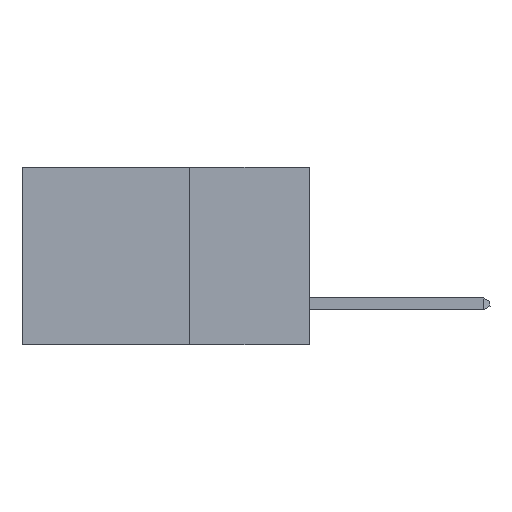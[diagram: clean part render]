
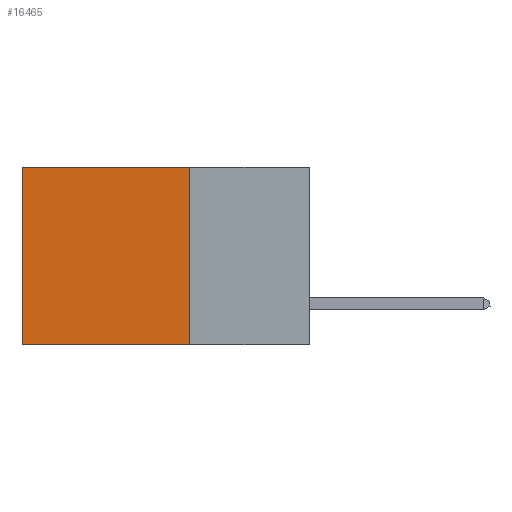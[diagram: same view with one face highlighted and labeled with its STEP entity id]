
A CAD part, left-side view. The second image highlights one B-rep face of the part: STEP entity #16465.
In plain terms, the highlighted planar face has unit normal (-1, 0, 0).
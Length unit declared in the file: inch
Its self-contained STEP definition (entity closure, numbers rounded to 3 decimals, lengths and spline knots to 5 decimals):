
#1023 = PLANE ( 'NONE',  #18464 ) ;
#1770 = CARTESIAN_POINT ( 'NONE',  ( 0.2875, 0.25, -0.37 ) ) ;
#1894 = VECTOR ( 'NONE', #9002, 39.37008 ) ;
#2197 = VECTOR ( 'NONE', #21519, 39.37008 ) ;
#2782 = ORIENTED_EDGE ( 'NONE', *, *, #11449, .T. ) ;
#3236 = DIRECTION ( 'NONE',  ( 1., 0., 0. ) ) ;
#3299 = EDGE_CURVE ( 'NONE', #24314, #27592, #8039, .T. ) ;
#4627 = VECTOR ( 'NONE', #26613, 39.37008 ) ;
#5849 = VERTEX_POINT ( 'NONE', #18993 ) ;
#7018 = FACE_OUTER_BOUND ( 'NONE', #21421, .T. ) ;
#7144 = LINE ( 'NONE', #16800, #16586 ) ;
#7405 = EDGE_CURVE ( 'NONE', #14922, #24314, #8406, .T. ) ;
#8039 = LINE ( 'NONE', #26032, #2197 ) ;
#8406 = LINE ( 'NONE', #21928, #1894 ) ;
#9002 = DIRECTION ( 'NONE',  ( 0., 0., -1. ) ) ;
#11449 = EDGE_CURVE ( 'NONE', #14922, #5849, #7144, .T. ) ;
#14922 = VERTEX_POINT ( 'NONE', #22315 ) ;
#16465 = ADVANCED_FACE ( 'NONE', ( #7018 ), #1023, .F. ) ;
#16586 = VECTOR ( 'NONE', #25249, 39.37008 ) ;
#16800 = CARTESIAN_POINT ( 'NONE',  ( 0.2875, 0.25, 0. ) ) ;
#17854 = CARTESIAN_POINT ( 'NONE',  ( 0.2875, 0.6, -0.37 ) ) ;
#18156 = LINE ( 'NONE', #24466, #4627 ) ;
#18367 = DIRECTION ( 'NONE',  ( 0., 0., -1. ) ) ;
#18464 = AXIS2_PLACEMENT_3D ( 'NONE', #26833, #3236, #18367 ) ;
#18905 = ORIENTED_EDGE ( 'NONE', *, *, #7405, .F. ) ;
#18993 = CARTESIAN_POINT ( 'NONE',  ( 0.2875, 0.6, 0. ) ) ;
#20200 = EDGE_CURVE ( 'NONE', #5849, #27592, #18156, .T. ) ;
#21421 = EDGE_LOOP ( 'NONE', ( #27409, #25983, #18905, #2782 ) ) ;
#21519 = DIRECTION ( 'NONE',  ( 0., 1., 0. ) ) ;
#21928 = CARTESIAN_POINT ( 'NONE',  ( 0.2875, 0.25, 0. ) ) ;
#22315 = CARTESIAN_POINT ( 'NONE',  ( 0.2875, 0.25, 0. ) ) ;
#24314 = VERTEX_POINT ( 'NONE', #1770 ) ;
#24466 = CARTESIAN_POINT ( 'NONE',  ( 0.2875, 0.6, 0. ) ) ;
#25249 = DIRECTION ( 'NONE',  ( 0., 1., 0. ) ) ;
#25983 = ORIENTED_EDGE ( 'NONE', *, *, #3299, .F. ) ;
#26032 = CARTESIAN_POINT ( 'NONE',  ( 0.2875, 0.25, -0.37 ) ) ;
#26613 = DIRECTION ( 'NONE',  ( 0., 0., -1. ) ) ;
#26833 = CARTESIAN_POINT ( 'NONE',  ( 0.2875, 0.25, 0. ) ) ;
#27409 = ORIENTED_EDGE ( 'NONE', *, *, #20200, .T. ) ;
#27592 = VERTEX_POINT ( 'NONE', #17854 ) ;
